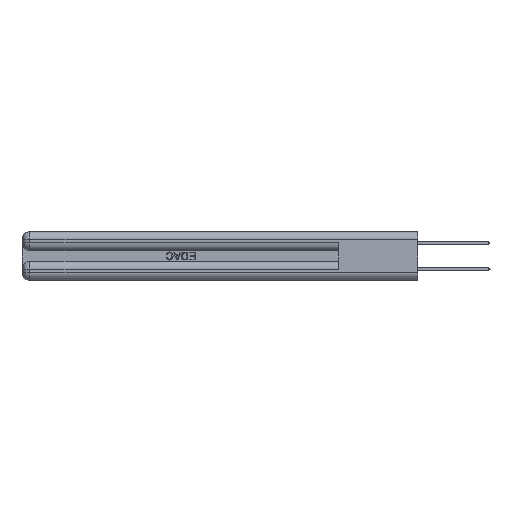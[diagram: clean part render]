
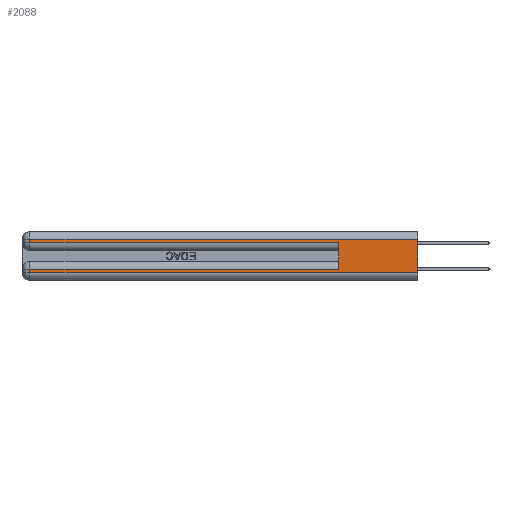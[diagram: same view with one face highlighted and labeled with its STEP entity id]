
A CAD part, left-side view. The second image highlights one B-rep face of the part: STEP entity #2088.
In plain terms, the highlighted planar face has unit normal (-1, 0, 0).
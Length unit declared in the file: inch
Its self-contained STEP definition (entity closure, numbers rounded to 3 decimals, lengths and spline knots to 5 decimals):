
#198 = CARTESIAN_POINT ( 'NONE',  ( 0., 0., 0.085 ) ) ;
#386 = LINE ( 'NONE', #13888, #45370 ) ;
#598 = CARTESIAN_POINT ( 'NONE',  ( 0., 0.6, 0.085 ) ) ;
#774 = PLANE ( 'NONE',  #21008 ) ;
#972 = DIRECTION ( 'NONE',  ( 0., -1., 0. ) ) ;
#1459 = CARTESIAN_POINT ( 'NONE',  ( 0., 0.6, 0.145 ) ) ;
#1678 = LINE ( 'NONE', #16902, #38371 ) ;
#2088 = ADVANCED_FACE ( 'NONE', ( #17255 ), #774, .F. ) ;
#2194 = CARTESIAN_POINT ( 'NONE',  ( 0., 0., 0.31 ) ) ;
#2953 = DIRECTION ( 'NONE',  ( 0., 0., -1. ) ) ;
#3579 = DIRECTION ( 'NONE',  ( 0., 0., -1. ) ) ;
#4104 = LINE ( 'NONE', #2194, #29096 ) ;
#4131 = CARTESIAN_POINT ( 'NONE',  ( 0., 2.94, 0.06 ) ) ;
#4175 = VECTOR ( 'NONE', #2953, 39.37008 ) ;
#4297 = EDGE_CURVE ( 'NONE', #14529, #28768, #22712, .T. ) ;
#6411 = EDGE_LOOP ( 'NONE', ( #12180, #40512, #24934, #7189, #35497, #37744, #10525, #23278 ) ) ;
#6835 = EDGE_CURVE ( 'NONE', #24597, #15160, #23028, .T. ) ;
#7189 = ORIENTED_EDGE ( 'NONE', *, *, #13280, .T. ) ;
#7734 = VERTEX_POINT ( 'NONE', #4131 ) ;
#7811 = LINE ( 'NONE', #35531, #14990 ) ;
#7932 = DIRECTION ( 'NONE',  ( 1., 0., 0. ) ) ;
#10483 = DIRECTION ( 'NONE',  ( 0., -1., 0. ) ) ;
#10525 = ORIENTED_EDGE ( 'NONE', *, *, #19375, .T. ) ;
#10917 = DIRECTION ( 'NONE',  ( 0., 1., 0. ) ) ;
#11304 = CARTESIAN_POINT ( 'NONE',  ( 0., 0.6, 0.285 ) ) ;
#12180 = ORIENTED_EDGE ( 'NONE', *, *, #6835, .F. ) ;
#12646 = CARTESIAN_POINT ( 'NONE',  ( 0., 2.94, 0.085 ) ) ;
#13280 = EDGE_CURVE ( 'NONE', #13796, #28768, #386, .T. ) ;
#13312 = VECTOR ( 'NONE', #44149, 39.37008 ) ;
#13796 = VERTEX_POINT ( 'NONE', #42276 ) ;
#13888 = CARTESIAN_POINT ( 'NONE',  ( 0., 0., 0.285 ) ) ;
#13943 = LINE ( 'NONE', #39962, #31724 ) ;
#14529 = VERTEX_POINT ( 'NONE', #598 ) ;
#14990 = VECTOR ( 'NONE', #3579, 39.37008 ) ;
#15160 = VERTEX_POINT ( 'NONE', #17884 ) ;
#16902 = CARTESIAN_POINT ( 'NONE',  ( 0., 2.94, 0.37 ) ) ;
#17255 = FACE_OUTER_BOUND ( 'NONE', #6411, .T. ) ;
#17884 = CARTESIAN_POINT ( 'NONE',  ( 0., 0., 0.06 ) ) ;
#19375 = EDGE_CURVE ( 'NONE', #37166, #7734, #1678, .T. ) ;
#19508 = EDGE_CURVE ( 'NONE', #29176, #13796, #7811, .T. ) ;
#21008 = AXIS2_PLACEMENT_3D ( 'NONE', #29190, #7932, #32755 ) ;
#22712 = LINE ( 'NONE', #1459, #13312 ) ;
#23028 = LINE ( 'NONE', #38362, #4175 ) ;
#23278 = ORIENTED_EDGE ( 'NONE', *, *, #32448, .T. ) ;
#23442 = DIRECTION ( 'NONE',  ( 0., 1., 0. ) ) ;
#24178 = CARTESIAN_POINT ( 'NONE',  ( 0., 0., 0.31 ) ) ;
#24597 = VERTEX_POINT ( 'NONE', #24178 ) ;
#24934 = ORIENTED_EDGE ( 'NONE', *, *, #19508, .T. ) ;
#28270 = VECTOR ( 'NONE', #10917, 39.37008 ) ;
#28768 = VERTEX_POINT ( 'NONE', #11304 ) ;
#29096 = VECTOR ( 'NONE', #23442, 39.37008 ) ;
#29176 = VERTEX_POINT ( 'NONE', #45398 ) ;
#29190 = CARTESIAN_POINT ( 'NONE',  ( 0., 0., 0.37 ) ) ;
#29385 = LINE ( 'NONE', #198, #28270 ) ;
#30880 = EDGE_CURVE ( 'NONE', #24597, #29176, #4104, .T. ) ;
#31724 = VECTOR ( 'NONE', #972, 39.37008 ) ;
#32448 = EDGE_CURVE ( 'NONE', #7734, #15160, #13943, .T. ) ;
#32755 = DIRECTION ( 'NONE',  ( 0., 0., -1. ) ) ;
#35497 = ORIENTED_EDGE ( 'NONE', *, *, #4297, .F. ) ;
#35531 = CARTESIAN_POINT ( 'NONE',  ( 0., 2.94, 0.37 ) ) ;
#37166 = VERTEX_POINT ( 'NONE', #12646 ) ;
#37552 = EDGE_CURVE ( 'NONE', #14529, #37166, #29385, .T. ) ;
#37744 = ORIENTED_EDGE ( 'NONE', *, *, #37552, .T. ) ;
#38362 = CARTESIAN_POINT ( 'NONE',  ( 0., 0., 0.37 ) ) ;
#38371 = VECTOR ( 'NONE', #41933, 39.37008 ) ;
#39962 = CARTESIAN_POINT ( 'NONE',  ( 0., 0., 0.06 ) ) ;
#40512 = ORIENTED_EDGE ( 'NONE', *, *, #30880, .T. ) ;
#41933 = DIRECTION ( 'NONE',  ( 0., 0., -1. ) ) ;
#42276 = CARTESIAN_POINT ( 'NONE',  ( 0., 2.94, 0.285 ) ) ;
#44149 = DIRECTION ( 'NONE',  ( 0., 0., 1. ) ) ;
#45370 = VECTOR ( 'NONE', #10483, 39.37008 ) ;
#45398 = CARTESIAN_POINT ( 'NONE',  ( 0., 2.94, 0.31 ) ) ;
